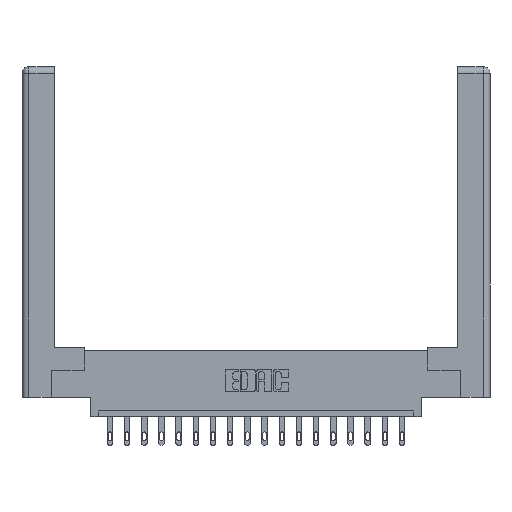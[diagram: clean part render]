
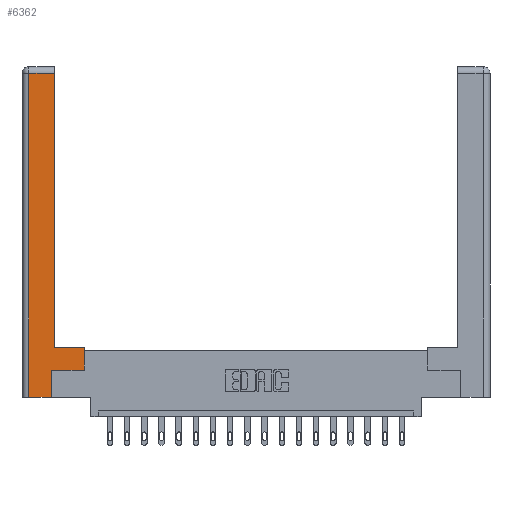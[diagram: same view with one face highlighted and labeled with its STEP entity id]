
A CAD part, top view. The second image highlights one B-rep face of the part: STEP entity #6362.
In plain terms, the highlighted planar face has unit normal (0, 0, 1).
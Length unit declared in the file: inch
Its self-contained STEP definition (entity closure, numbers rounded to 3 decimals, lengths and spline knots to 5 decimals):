
#131 = VECTOR ( 'NONE', #13362, 39.37008 ) ;
#140 = CARTESIAN_POINT ( 'NONE',  ( 0.265, 0., 0. ) ) ;
#237 = DIRECTION ( 'NONE',  ( 0., 1., 0. ) ) ;
#249 = CARTESIAN_POINT ( 'NONE',  ( 0.0615, 2.94, 0. ) ) ;
#260 = ORIENTED_EDGE ( 'NONE', *, *, #11441, .T. ) ;
#303 = CARTESIAN_POINT ( 'NONE',  ( 0.295, 2.94, 0. ) ) ;
#621 = DIRECTION ( 'NONE',  ( 0., 1., 0. ) ) ;
#867 = CARTESIAN_POINT ( 'NONE',  ( 0., 0., 0. ) ) ;
#1162 = DIRECTION ( 'NONE',  ( -1., 0., 0. ) ) ;
#1223 = LINE ( 'NONE', #12539, #16273 ) ;
#1354 = CARTESIAN_POINT ( 'NONE',  ( 0.265, 0., 0. ) ) ;
#1826 = ORIENTED_EDGE ( 'NONE', *, *, #17886, .T. ) ;
#3262 = VECTOR ( 'NONE', #621, 39.37008 ) ;
#3366 = AXIS2_PLACEMENT_3D ( 'NONE', #867, #14260, #15732 ) ;
#4558 = CARTESIAN_POINT ( 'NONE',  ( 0.265, 0.245, 0. ) ) ;
#5554 = EDGE_CURVE ( 'NONE', #16851, #12941, #12379, .T. ) ;
#6362 = ADVANCED_FACE ( 'NONE', ( #10555 ), #14137, .F. ) ;
#6422 = CARTESIAN_POINT ( 'NONE',  ( 0.565, 0.45, 0. ) ) ;
#6453 = ORIENTED_EDGE ( 'NONE', *, *, #16535, .T. ) ;
#6829 = ORIENTED_EDGE ( 'NONE', *, *, #9726, .T. ) ;
#7093 = VECTOR ( 'NONE', #237, 39.37008 ) ;
#7217 = EDGE_CURVE ( 'NONE', #13702, #9625, #11312, .T. ) ;
#7417 = CARTESIAN_POINT ( 'NONE',  ( 0.295, 0.45, 0. ) ) ;
#7425 = VERTEX_POINT ( 'NONE', #249 ) ;
#7749 = VECTOR ( 'NONE', #16405, 39.37008 ) ;
#8166 = ORIENTED_EDGE ( 'NONE', *, *, #17502, .T. ) ;
#8188 = CARTESIAN_POINT ( 'NONE',  ( 0.565, 0.245, 0. ) ) ;
#8559 = CARTESIAN_POINT ( 'NONE',  ( 0.295, 0.45, 0. ) ) ;
#8777 = VECTOR ( 'NONE', #9691, 39.37008 ) ;
#9149 = CARTESIAN_POINT ( 'NONE',  ( 0.565, 0.45, 0. ) ) ;
#9625 = VERTEX_POINT ( 'NONE', #16269 ) ;
#9691 = DIRECTION ( 'NONE',  ( 1., 0., 0. ) ) ;
#9726 = EDGE_CURVE ( 'NONE', #13726, #13702, #16548, .T. ) ;
#10118 = LINE ( 'NONE', #9149, #7093 ) ;
#10322 = EDGE_CURVE ( 'NONE', #16786, #7425, #1223, .T. ) ;
#10555 = FACE_OUTER_BOUND ( 'NONE', #18358, .T. ) ;
#11214 = CARTESIAN_POINT ( 'NONE',  ( 0.295, 3., 0. ) ) ;
#11312 = LINE ( 'NONE', #8188, #8777 ) ;
#11441 = EDGE_CURVE ( 'NONE', #7425, #12251, #18088, .T. ) ;
#11509 = LINE ( 'NONE', #140, #12213 ) ;
#12213 = VECTOR ( 'NONE', #19176, 39.37008 ) ;
#12251 = VERTEX_POINT ( 'NONE', #17237 ) ;
#12379 = LINE ( 'NONE', #7417, #131 ) ;
#12539 = CARTESIAN_POINT ( 'NONE',  ( 0.0615, 2.94, 0. ) ) ;
#12694 = LINE ( 'NONE', #11214, #3262 ) ;
#12816 = ORIENTED_EDGE ( 'NONE', *, *, #5554, .T. ) ;
#12941 = VERTEX_POINT ( 'NONE', #8559 ) ;
#13362 = DIRECTION ( 'NONE',  ( -1., 0., 0. ) ) ;
#13702 = VERTEX_POINT ( 'NONE', #18634 ) ;
#13726 = VERTEX_POINT ( 'NONE', #1354 ) ;
#13959 = CARTESIAN_POINT ( 'NONE',  ( 0.0615, 0., 0. ) ) ;
#14137 = PLANE ( 'NONE',  #3366 ) ;
#14260 = DIRECTION ( 'NONE',  ( 0., 0., -1. ) ) ;
#15424 = DIRECTION ( 'NONE',  ( 0., -1., 0. ) ) ;
#15732 = DIRECTION ( 'NONE',  ( -1., 0., 0. ) ) ;
#15966 = ORIENTED_EDGE ( 'NONE', *, *, #7217, .T. ) ;
#16269 = CARTESIAN_POINT ( 'NONE',  ( 0.565, 0.245, 0. ) ) ;
#16273 = VECTOR ( 'NONE', #1162, 39.37008 ) ;
#16405 = DIRECTION ( 'NONE',  ( 0., 1., 0. ) ) ;
#16535 = EDGE_CURVE ( 'NONE', #12941, #16786, #12694, .T. ) ;
#16548 = LINE ( 'NONE', #4558, #7749 ) ;
#16786 = VERTEX_POINT ( 'NONE', #303 ) ;
#16851 = VERTEX_POINT ( 'NONE', #6422 ) ;
#17237 = CARTESIAN_POINT ( 'NONE',  ( 0.0615, 0., 0. ) ) ;
#17400 = VECTOR ( 'NONE', #15424, 39.37008 ) ;
#17502 = EDGE_CURVE ( 'NONE', #12251, #13726, #11509, .T. ) ;
#17886 = EDGE_CURVE ( 'NONE', #9625, #16851, #10118, .T. ) ;
#18088 = LINE ( 'NONE', #13959, #17400 ) ;
#18358 = EDGE_LOOP ( 'NONE', ( #6453, #18365, #260, #8166, #6829, #15966, #1826, #12816 ) ) ;
#18365 = ORIENTED_EDGE ( 'NONE', *, *, #10322, .T. ) ;
#18634 = CARTESIAN_POINT ( 'NONE',  ( 0.265, 0.245, 0. ) ) ;
#19176 = DIRECTION ( 'NONE',  ( 1., 0., 0. ) ) ;
